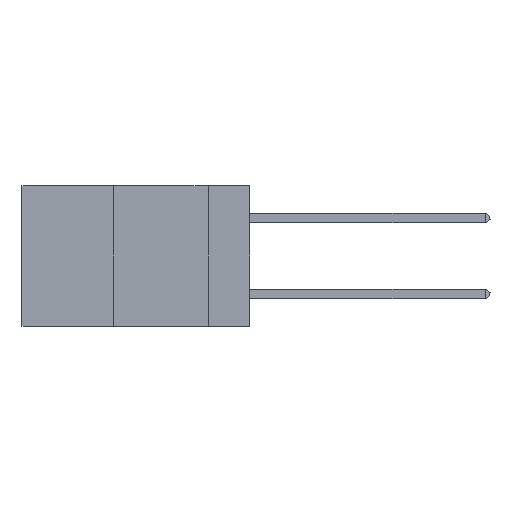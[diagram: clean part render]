
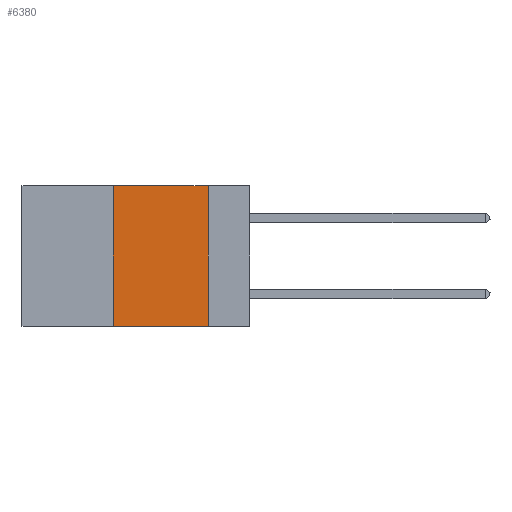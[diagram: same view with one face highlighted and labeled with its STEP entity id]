
A CAD part, left-side view. The second image highlights one B-rep face of the part: STEP entity #6380.
In plain terms, the highlighted planar face has unit normal (-1, 0, 0).
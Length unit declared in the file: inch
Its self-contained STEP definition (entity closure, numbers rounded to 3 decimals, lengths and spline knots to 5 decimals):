
#139 = DIRECTION ( 'NONE',  ( 1., 0., 0. ) ) ;
#668 = CARTESIAN_POINT ( 'NONE',  ( 0., 0.11, 0. ) ) ;
#729 = CARTESIAN_POINT ( 'NONE',  ( 0., 0.11, 0. ) ) ;
#1227 = LINE ( 'NONE', #668, #5731 ) ;
#1273 = DIRECTION ( 'NONE',  ( 0., -1., 0. ) ) ;
#1301 = AXIS2_PLACEMENT_3D ( 'NONE', #4816, #139, #13179 ) ;
#2476 = EDGE_CURVE ( 'NONE', #2647, #13925, #15218, .T. ) ;
#2529 = EDGE_CURVE ( 'NONE', #4172, #13925, #1227, .T. ) ;
#2647 = VERTEX_POINT ( 'NONE', #8930 ) ;
#2727 = EDGE_CURVE ( 'NONE', #2647, #9250, #5363, .T. ) ;
#3178 = DIRECTION ( 'NONE',  ( 0., 0., 1. ) ) ;
#4172 = VERTEX_POINT ( 'NONE', #729 ) ;
#4229 = DIRECTION ( 'NONE',  ( 0., 0., -1. ) ) ;
#4438 = CARTESIAN_POINT ( 'NONE',  ( 0., 0.36, 0. ) ) ;
#4681 = CARTESIAN_POINT ( 'NONE',  ( 0., 0.6, 0. ) ) ;
#4816 = CARTESIAN_POINT ( 'NONE',  ( 0., 0.6, 0. ) ) ;
#4829 = ORIENTED_EDGE ( 'NONE', *, *, #2529, .F. ) ;
#5363 = LINE ( 'NONE', #4438, #9265 ) ;
#5731 = VECTOR ( 'NONE', #4229, 39.37008 ) ;
#5737 = CARTESIAN_POINT ( 'NONE',  ( 0., 0.36, 0. ) ) ;
#5782 = VECTOR ( 'NONE', #1273, 39.37008 ) ;
#6231 = CARTESIAN_POINT ( 'NONE',  ( 0., 0.6, -0.37 ) ) ;
#6380 = ADVANCED_FACE ( 'NONE', ( #12776 ), #7314, .F. ) ;
#7314 = PLANE ( 'NONE',  #1301 ) ;
#7961 = VECTOR ( 'NONE', #8766, 39.37008 ) ;
#8766 = DIRECTION ( 'NONE',  ( 0., -1., 0. ) ) ;
#8930 = CARTESIAN_POINT ( 'NONE',  ( 0., 0.36, -0.37 ) ) ;
#8954 = LINE ( 'NONE', #4681, #5782 ) ;
#9250 = VERTEX_POINT ( 'NONE', #5737 ) ;
#9265 = VECTOR ( 'NONE', #3178, 39.37008 ) ;
#9395 = EDGE_LOOP ( 'NONE', ( #4829, #10089, #14792, #9633 ) ) ;
#9633 = ORIENTED_EDGE ( 'NONE', *, *, #2476, .T. ) ;
#10089 = ORIENTED_EDGE ( 'NONE', *, *, #10208, .F. ) ;
#10208 = EDGE_CURVE ( 'NONE', #9250, #4172, #8954, .T. ) ;
#12776 = FACE_OUTER_BOUND ( 'NONE', #9395, .T. ) ;
#13179 = DIRECTION ( 'NONE',  ( 0., 0., -1. ) ) ;
#13546 = CARTESIAN_POINT ( 'NONE',  ( 0., 0.11, -0.37 ) ) ;
#13925 = VERTEX_POINT ( 'NONE', #13546 ) ;
#14792 = ORIENTED_EDGE ( 'NONE', *, *, #2727, .F. ) ;
#15218 = LINE ( 'NONE', #6231, #7961 ) ;
